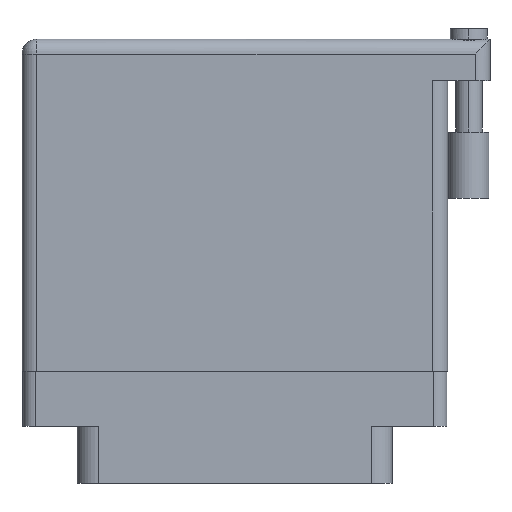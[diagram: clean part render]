
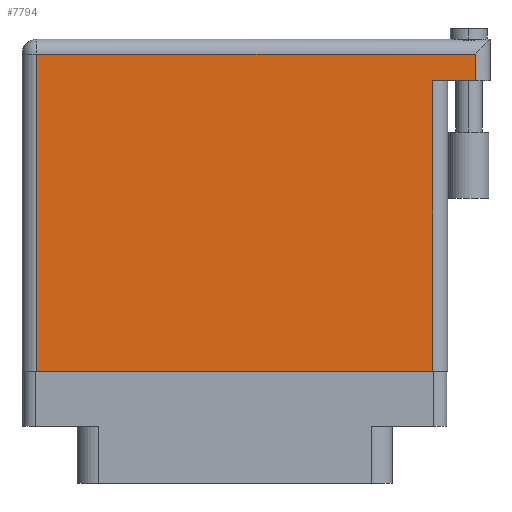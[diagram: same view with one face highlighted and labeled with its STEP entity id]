
A CAD part, front view. The second image highlights one B-rep face of the part: STEP entity #7794.
In plain terms, the highlighted face is planar.
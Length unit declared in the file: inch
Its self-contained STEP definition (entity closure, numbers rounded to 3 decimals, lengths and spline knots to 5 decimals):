
#301 = CARTESIAN_POINT ( 'NONE',  ( 0., 1.496, 0. ) ) ;
#1035 = DIRECTION ( 'NONE',  ( 0., 0., -1. ) ) ;
#1282 = LINE ( 'NONE', #4736, #24595 ) ;
#1590 = EDGE_CURVE ( 'NONE', #34088, #17433, #3034, .T. ) ;
#2100 = LINE ( 'NONE', #301, #24937 ) ;
#3034 = LINE ( 'NONE', #23628, #31511 ) ;
#3511 = CARTESIAN_POINT ( 'NONE',  ( 2.208, 1.369, 0. ) ) ;
#4736 = CARTESIAN_POINT ( 'NONE',  ( 2.138, 1.566, 0. ) ) ;
#6466 = CARTESIAN_POINT ( 'NONE',  ( 1.938, 1.369, 0. ) ) ;
#6991 = ORIENTED_EDGE ( 'NONE', *, *, #1590, .T. ) ;
#7752 = CARTESIAN_POINT ( 'NONE',  ( 1.938, 1.369, 0. ) ) ;
#7794 = ADVANCED_FACE ( 'NONE', ( #34316 ), #21622, .F. ) ;
#8389 = VERTEX_POINT ( 'NONE', #36123 ) ;
#8675 = ORIENTED_EDGE ( 'NONE', *, *, #36165, .F. ) ;
#12101 = DIRECTION ( 'NONE',  ( -1., 0., 0. ) ) ;
#12855 = DIRECTION ( 'NONE',  ( 0., -1., 0. ) ) ;
#14177 = EDGE_CURVE ( 'NONE', #8389, #19732, #2100, .T. ) ;
#15050 = VECTOR ( 'NONE', #33497, 39.37008 ) ;
#16574 = VERTEX_POINT ( 'NONE', #20776 ) ;
#17433 = VERTEX_POINT ( 'NONE', #33504 ) ;
#18527 = EDGE_CURVE ( 'NONE', #16574, #8389, #1282, .T. ) ;
#18591 = CARTESIAN_POINT ( 'NONE',  ( 0.07, 0., 0. ) ) ;
#19676 = CARTESIAN_POINT ( 'NONE',  ( 0.07, 1.496, 0. ) ) ;
#19732 = VERTEX_POINT ( 'NONE', #19676 ) ;
#19864 = LINE ( 'NONE', #18591, #32529 ) ;
#20395 = CARTESIAN_POINT ( 'NONE',  ( 0.07, 0., 0. ) ) ;
#20776 = CARTESIAN_POINT ( 'NONE',  ( 2.138, 1.369, 0. ) ) ;
#21282 = AXIS2_PLACEMENT_3D ( 'NONE', #36802, #1035, #33653 ) ;
#21531 = ORIENTED_EDGE ( 'NONE', *, *, #14177, .T. ) ;
#21622 = PLANE ( 'NONE',  #21282 ) ;
#22719 = EDGE_CURVE ( 'NONE', #17433, #22891, #38376, .T. ) ;
#22891 = VERTEX_POINT ( 'NONE', #7752 ) ;
#23628 = CARTESIAN_POINT ( 'NONE',  ( 0., 0., 0. ) ) ;
#24157 = VECTOR ( 'NONE', #12101, 39.37008 ) ;
#24595 = VECTOR ( 'NONE', #25736, 39.37008 ) ;
#24937 = VECTOR ( 'NONE', #27046, 39.37008 ) ;
#25736 = DIRECTION ( 'NONE',  ( 0., 1., 0. ) ) ;
#27046 = DIRECTION ( 'NONE',  ( -1., 0., 0. ) ) ;
#27623 = ORIENTED_EDGE ( 'NONE', *, *, #18527, .T. ) ;
#28341 = EDGE_CURVE ( 'NONE', #19732, #34088, #19864, .T. ) ;
#29479 = EDGE_LOOP ( 'NONE', ( #6991, #37903, #8675, #27623, #21531, #33054 ) ) ;
#29859 = LINE ( 'NONE', #3511, #24157 ) ;
#31511 = VECTOR ( 'NONE', #32258, 39.37008 ) ;
#32258 = DIRECTION ( 'NONE',  ( 1., 0., 0. ) ) ;
#32529 = VECTOR ( 'NONE', #12855, 39.37008 ) ;
#33054 = ORIENTED_EDGE ( 'NONE', *, *, #28341, .T. ) ;
#33497 = DIRECTION ( 'NONE',  ( 0., 1., 0. ) ) ;
#33504 = CARTESIAN_POINT ( 'NONE',  ( 1.938, 0., 0. ) ) ;
#33653 = DIRECTION ( 'NONE',  ( -1., 0., 0. ) ) ;
#34088 = VERTEX_POINT ( 'NONE', #20395 ) ;
#34316 = FACE_OUTER_BOUND ( 'NONE', #29479, .T. ) ;
#36123 = CARTESIAN_POINT ( 'NONE',  ( 2.138, 1.496, 0. ) ) ;
#36165 = EDGE_CURVE ( 'NONE', #16574, #22891, #29859, .T. ) ;
#36802 = CARTESIAN_POINT ( 'NONE',  ( 0., 1.566, 0. ) ) ;
#37903 = ORIENTED_EDGE ( 'NONE', *, *, #22719, .T. ) ;
#38376 = LINE ( 'NONE', #6466, #15050 ) ;
